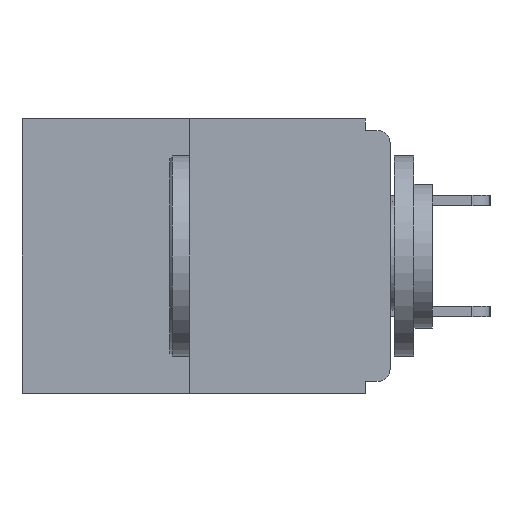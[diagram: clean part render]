
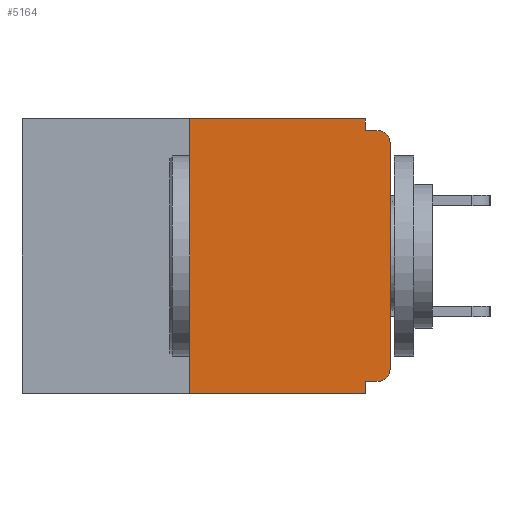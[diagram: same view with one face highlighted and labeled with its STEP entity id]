
A CAD part, left-side view. The second image highlights one B-rep face of the part: STEP entity #5164.
In plain terms, the highlighted planar face has unit normal (-1, 0, 0).
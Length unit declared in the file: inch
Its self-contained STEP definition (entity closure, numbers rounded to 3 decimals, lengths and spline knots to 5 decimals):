
#208 = VECTOR ( 'NONE', #8005, 39.37008 ) ;
#585 = FACE_OUTER_BOUND ( 'NONE', #5727, .T. ) ;
#588 = CARTESIAN_POINT ( 'NONE',  ( 0., 0.031, 0. ) ) ;
#798 = VERTEX_POINT ( 'NONE', #2060 ) ;
#969 = VECTOR ( 'NONE', #5236, 39.37008 ) ;
#1335 = DIRECTION ( 'NONE',  ( 0., 0., 1. ) ) ;
#1340 = CARTESIAN_POINT ( 'NONE',  ( 0., 0.25, 0. ) ) ;
#1393 = VERTEX_POINT ( 'NONE', #11612 ) ;
#1650 = CARTESIAN_POINT ( 'NONE',  ( 0., 0., -0.328 ) ) ;
#1674 = VECTOR ( 'NONE', #7211, 39.37008 ) ;
#1878 = ORIENTED_EDGE ( 'NONE', *, *, #10801, .F. ) ;
#2060 = CARTESIAN_POINT ( 'NONE',  ( 0., 0., -0.03 ) ) ;
#2088 = VERTEX_POINT ( 'NONE', #12507 ) ;
#2157 = DIRECTION ( 'NONE',  ( 0., 0., -1. ) ) ;
#2300 = VECTOR ( 'NONE', #1335, 39.37008 ) ;
#2359 = CARTESIAN_POINT ( 'NONE',  ( 0., 0., -0.015 ) ) ;
#2374 = CARTESIAN_POINT ( 'NONE',  ( 0., 0.46, 0. ) ) ;
#2476 = AXIS2_PLACEMENT_3D ( 'NONE', #9075, #12032, #9992 ) ;
#2556 = VECTOR ( 'NONE', #4342, 39.37008 ) ;
#2713 = AXIS2_PLACEMENT_3D ( 'NONE', #6111, #8096, #2157 ) ;
#2788 = EDGE_CURVE ( 'NONE', #798, #9327, #6968, .T. ) ;
#2814 = ORIENTED_EDGE ( 'NONE', *, *, #12624, .F. ) ;
#3263 = ORIENTED_EDGE ( 'NONE', *, *, #9065, .F. ) ;
#3293 = CARTESIAN_POINT ( 'NONE',  ( 0., 0., 0. ) ) ;
#3346 = ORIENTED_EDGE ( 'NONE', *, *, #12144, .T. ) ;
#3394 = DIRECTION ( 'NONE',  ( 0., -1., 0. ) ) ;
#3592 = VECTOR ( 'NONE', #5531, 39.37008 ) ;
#3793 = VERTEX_POINT ( 'NONE', #5129 ) ;
#3795 = LINE ( 'NONE', #10417, #2556 ) ;
#3821 = VECTOR ( 'NONE', #3394, 39.37008 ) ;
#3938 = ORIENTED_EDGE ( 'NONE', *, *, #2788, .T. ) ;
#4342 = DIRECTION ( 'NONE',  ( 0., 0., -1. ) ) ;
#4467 = CIRCLE ( 'NONE', #9046, 0.015 ) ;
#4591 = DIRECTION ( 'NONE',  ( 0., 0., -1. ) ) ;
#4856 = ORIENTED_EDGE ( 'NONE', *, *, #11134, .F. ) ;
#4893 = LINE ( 'NONE', #2359, #3821 ) ;
#5042 = ORIENTED_EDGE ( 'NONE', *, *, #9624, .F. ) ;
#5129 = CARTESIAN_POINT ( 'NONE',  ( 0., 0.031, -0.343 ) ) ;
#5164 = ADVANCED_FACE ( 'NONE', ( #585 ), #11099, .F. ) ;
#5236 = DIRECTION ( 'NONE',  ( 0., 0., 1. ) ) ;
#5426 = VECTOR ( 'NONE', #11699, 39.37008 ) ;
#5531 = DIRECTION ( 'NONE',  ( 0., -1., 0. ) ) ;
#5623 = LINE ( 'NONE', #6526, #3592 ) ;
#5727 = EDGE_LOOP ( 'NONE', ( #2814, #1878, #9998, #4856, #5042, #3346, #12672, #3938, #8771, #3263 ) ) ;
#5828 = VERTEX_POINT ( 'NONE', #9262 ) ;
#5881 = LINE ( 'NONE', #3293, #2300 ) ;
#5900 = EDGE_CURVE ( 'NONE', #11855, #9327, #4893, .T. ) ;
#6111 = CARTESIAN_POINT ( 'NONE',  ( 0., 0.015, -0.03 ) ) ;
#6526 = CARTESIAN_POINT ( 'NONE',  ( 0., 0.46, -0.343 ) ) ;
#6710 = DIRECTION ( 'NONE',  ( -1., 0., 0. ) ) ;
#6797 = VERTEX_POINT ( 'NONE', #10761 ) ;
#6968 = CIRCLE ( 'NONE', #2713, 0.015 ) ;
#6973 = CARTESIAN_POINT ( 'NONE',  ( 0., 0.031, -0.015 ) ) ;
#7211 = DIRECTION ( 'NONE',  ( 0., -1., 0. ) ) ;
#8005 = DIRECTION ( 'NONE',  ( 0., 1., 0. ) ) ;
#8064 = LINE ( 'NONE', #10717, #5426 ) ;
#8096 = DIRECTION ( 'NONE',  ( -1., 0., 0. ) ) ;
#8146 = VERTEX_POINT ( 'NONE', #588 ) ;
#8771 = ORIENTED_EDGE ( 'NONE', *, *, #5900, .F. ) ;
#8892 = LINE ( 'NONE', #1340, #969 ) ;
#9046 = AXIS2_PLACEMENT_3D ( 'NONE', #10623, #6710, #4591 ) ;
#9065 = EDGE_CURVE ( 'NONE', #8146, #11855, #3795, .T. ) ;
#9075 = CARTESIAN_POINT ( 'NONE',  ( 0., 0.46, 0. ) ) ;
#9262 = CARTESIAN_POINT ( 'NONE',  ( 0., 0.25, 0. ) ) ;
#9283 = CARTESIAN_POINT ( 'NONE',  ( 0., 0.015, -0.015 ) ) ;
#9327 = VERTEX_POINT ( 'NONE', #9283 ) ;
#9609 = LINE ( 'NONE', #2374, #1674 ) ;
#9624 = EDGE_CURVE ( 'NONE', #1393, #2088, #11359, .T. ) ;
#9992 = DIRECTION ( 'NONE',  ( 0., 0., -1. ) ) ;
#9998 = ORIENTED_EDGE ( 'NONE', *, *, #10347, .T. ) ;
#10347 = EDGE_CURVE ( 'NONE', #6797, #3793, #5623, .T. ) ;
#10417 = CARTESIAN_POINT ( 'NONE',  ( 0., 0.031, 0. ) ) ;
#10623 = CARTESIAN_POINT ( 'NONE',  ( 0., 0.015, -0.313 ) ) ;
#10717 = CARTESIAN_POINT ( 'NONE',  ( 0., 0.031, -0.343 ) ) ;
#10761 = CARTESIAN_POINT ( 'NONE',  ( 0., 0.25, -0.343 ) ) ;
#10801 = EDGE_CURVE ( 'NONE', #6797, #5828, #8892, .T. ) ;
#11099 = PLANE ( 'NONE',  #2476 ) ;
#11134 = EDGE_CURVE ( 'NONE', #2088, #3793, #8064, .T. ) ;
#11359 = LINE ( 'NONE', #1650, #208 ) ;
#11612 = CARTESIAN_POINT ( 'NONE',  ( 0., 0.015, -0.328 ) ) ;
#11699 = DIRECTION ( 'NONE',  ( 0., 0., -1. ) ) ;
#11855 = VERTEX_POINT ( 'NONE', #6973 ) ;
#11943 = EDGE_CURVE ( 'NONE', #12696, #798, #5881, .T. ) ;
#12032 = DIRECTION ( 'NONE',  ( 1., 0., 0. ) ) ;
#12144 = EDGE_CURVE ( 'NONE', #1393, #12696, #4467, .T. ) ;
#12314 = CARTESIAN_POINT ( 'NONE',  ( 0., 0., -0.313 ) ) ;
#12507 = CARTESIAN_POINT ( 'NONE',  ( 0., 0.031, -0.328 ) ) ;
#12624 = EDGE_CURVE ( 'NONE', #5828, #8146, #9609, .T. ) ;
#12672 = ORIENTED_EDGE ( 'NONE', *, *, #11943, .T. ) ;
#12696 = VERTEX_POINT ( 'NONE', #12314 ) ;
